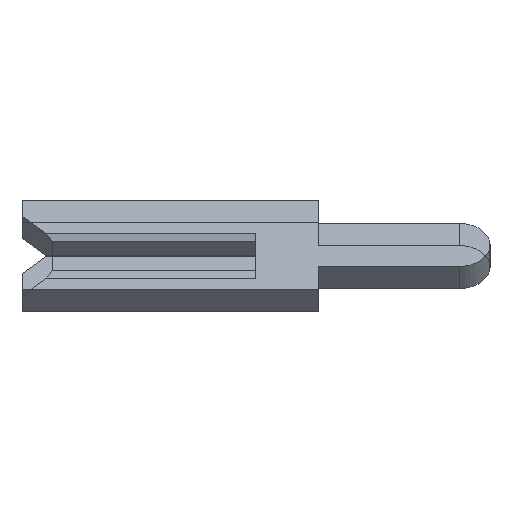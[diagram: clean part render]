
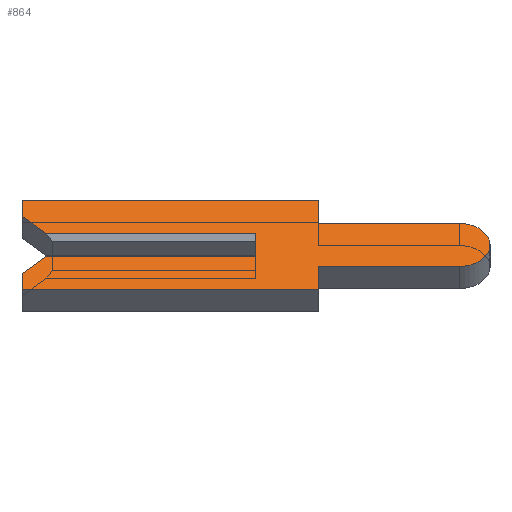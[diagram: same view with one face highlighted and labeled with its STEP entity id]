
A CAD part, left-side view. The second image highlights one B-rep face of the part: STEP entity #864.
In plain terms, the highlighted face is planar.
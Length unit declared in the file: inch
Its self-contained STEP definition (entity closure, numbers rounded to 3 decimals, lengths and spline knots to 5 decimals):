
#9 = CARTESIAN_POINT ( 'NONE',  ( -0.01, -0.1305, 0. ) ) ;
#24 = DIRECTION ( 'NONE',  ( 0., 0., -1. ) ) ;
#28 = VERTEX_POINT ( 'NONE', #462 ) ;
#91 = EDGE_CURVE ( 'NONE', #2926, #1471, #1673, .T. ) ;
#92 = CARTESIAN_POINT ( 'NONE',  ( -0.01, -0.04, 0.0195 ) ) ;
#119 = VECTOR ( 'NONE', #1464, 39.37008 ) ;
#138 = VECTOR ( 'NONE', #2182, 39.37008 ) ;
#164 = EDGE_CURVE ( 'NONE', #231, #1471, #1262, .T. ) ;
#183 = CARTESIAN_POINT ( 'NONE',  ( -0.01, 0.1305, -0.0065 ) ) ;
#231 = VERTEX_POINT ( 'NONE', #2669 ) ;
#281 = VERTEX_POINT ( 'NONE', #2938 ) ;
#291 = FACE_OUTER_BOUND ( 'NONE', #2627, .T. ) ;
#386 = ORIENTED_EDGE ( 'NONE', *, *, #2870, .F. ) ;
#456 = CARTESIAN_POINT ( 'NONE',  ( -0.01, 0.15, -0.026 ) ) ;
#462 = CARTESIAN_POINT ( 'NONE',  ( -0.01, -0.04, -0.0195 ) ) ;
#463 = EDGE_CURVE ( 'NONE', #2926, #2965, #843, .T. ) ;
#465 = VECTOR ( 'NONE', #735, 39.37008 ) ;
#523 = CARTESIAN_POINT ( 'NONE',  ( -0.01, 0., 0.0065 ) ) ;
#561 = DIRECTION ( 'NONE',  ( 1., 0., 0. ) ) ;
#573 = CARTESIAN_POINT ( 'NONE',  ( -0.01, -0.04, -0.04 ) ) ;
#591 = VECTOR ( 'NONE', #1389, 39.37008 ) ;
#613 = ORIENTED_EDGE ( 'NONE', *, *, #886, .F. ) ;
#616 = AXIS2_PLACEMENT_3D ( 'NONE', #9, #561, #24 ) ;
#646 = DIRECTION ( 'NONE',  ( 0., 0., -1. ) ) ;
#657 = CARTESIAN_POINT ( 'NONE',  ( -0.01, -0.1305, 0. ) ) ;
#684 = VERTEX_POINT ( 'NONE', #2724 ) ;
#710 = EDGE_CURVE ( 'NONE', #684, #231, #763, .T. ) ;
#728 = DIRECTION ( 'NONE',  ( 0., 0., 1. ) ) ;
#735 = DIRECTION ( 'NONE',  ( 0., -0.707, 0.707 ) ) ;
#763 = LINE ( 'NONE', #1929, #591 ) ;
#774 = ORIENTED_EDGE ( 'NONE', *, *, #2505, .F. ) ;
#800 = EDGE_CURVE ( 'NONE', #2965, #935, #2738, .T. ) ;
#820 = ORIENTED_EDGE ( 'NONE', *, *, #91, .T. ) ;
#829 = DIRECTION ( 'NONE',  ( 0., -1., 0. ) ) ;
#843 = LINE ( 'NONE', #2047, #138 ) ;
#864 = ADVANCED_FACE ( 'NONE', ( #291 ), #1636, .F. ) ;
#869 = VECTOR ( 'NONE', #1067, 39.37008 ) ;
#886 = EDGE_CURVE ( 'NONE', #1972, #3171, #2114, .T. ) ;
#935 = VERTEX_POINT ( 'NONE', #3116 ) ;
#1065 = VERTEX_POINT ( 'NONE', #3326 ) ;
#1067 = DIRECTION ( 'NONE',  ( 0., -1., 0. ) ) ;
#1164 = DIRECTION ( 'NONE',  ( 0., -1., 0. ) ) ;
#1177 = LINE ( 'NONE', #183, #465 ) ;
#1187 = EDGE_CURVE ( 'NONE', #28, #1530, #1839, .T. ) ;
#1262 = LINE ( 'NONE', #523, #1321 ) ;
#1277 = ORIENTED_EDGE ( 'NONE', *, *, #2949, .F. ) ;
#1303 = ORIENTED_EDGE ( 'NONE', *, *, #164, .F. ) ;
#1321 = VECTOR ( 'NONE', #1600, 39.37008 ) ;
#1327 = CARTESIAN_POINT ( 'NONE',  ( -0.01, 0.15, 0.01 ) ) ;
#1375 = CARTESIAN_POINT ( 'NONE',  ( -0.01, 0.15, 0.026 ) ) ;
#1389 = DIRECTION ( 'NONE',  ( 0., -1., 0. ) ) ;
#1464 = DIRECTION ( 'NONE',  ( 0., 1., 0. ) ) ;
#1471 = VERTEX_POINT ( 'NONE', #2883 ) ;
#1485 = ORIENTED_EDGE ( 'NONE', *, *, #1187, .F. ) ;
#1530 = VERTEX_POINT ( 'NONE', #2732 ) ;
#1557 = LINE ( 'NONE', #2789, #119 ) ;
#1561 = ORIENTED_EDGE ( 'NONE', *, *, #800, .F. ) ;
#1564 = CARTESIAN_POINT ( 'NONE',  ( -0.01, -0.1305, -0.0195 ) ) ;
#1573 = VECTOR ( 'NONE', #3124, 39.37008 ) ;
#1582 = LINE ( 'NONE', #456, #3179 ) ;
#1589 = VERTEX_POINT ( 'NONE', #1564 ) ;
#1600 = DIRECTION ( 'NONE',  ( 0., 0., 1. ) ) ;
#1636 = PLANE ( 'NONE',  #616 ) ;
#1673 = LINE ( 'NONE', #1327, #869 ) ;
#1768 = LINE ( 'NONE', #3133, #3098 ) ;
#1804 = EDGE_CURVE ( 'NONE', #281, #684, #1177, .T. ) ;
#1831 = ORIENTED_EDGE ( 'NONE', *, *, #2131, .F. ) ;
#1839 = LINE ( 'NONE', #573, #1573 ) ;
#1842 = VERTEX_POINT ( 'NONE', #2617 ) ;
#1852 = LINE ( 'NONE', #3298, #3362 ) ;
#1881 = CIRCLE ( 'NONE', #2850, 0.0195 ) ;
#1889 = EDGE_CURVE ( 'NONE', #3171, #1589, #1881, .T. ) ;
#1908 = CARTESIAN_POINT ( 'NONE',  ( -0.01, -0.04, 0.0195 ) ) ;
#1929 = CARTESIAN_POINT ( 'NONE',  ( -0.01, -0.1305, -0.01 ) ) ;
#1972 = VERTEX_POINT ( 'NONE', #92 ) ;
#2011 = CARTESIAN_POINT ( 'NONE',  ( -0.01, -0.1305, 0.0195 ) ) ;
#2047 = CARTESIAN_POINT ( 'NONE',  ( -0.01, 0.1305, 0.0065 ) ) ;
#2048 = ORIENTED_EDGE ( 'NONE', *, *, #463, .F. ) ;
#2094 = ORIENTED_EDGE ( 'NONE', *, *, #1889, .F. ) ;
#2114 = LINE ( 'NONE', #1908, #2187 ) ;
#2131 = EDGE_CURVE ( 'NONE', #1530, #1065, #1557, .T. ) ;
#2182 = DIRECTION ( 'NONE',  ( 0., 0.707, 0.707 ) ) ;
#2187 = VECTOR ( 'NONE', #829, 39.37008 ) ;
#2246 = DIRECTION ( 'NONE',  ( 1., 0., 0. ) ) ;
#2254 = CARTESIAN_POINT ( 'NONE',  ( -0.01, -0.04, 0.04 ) ) ;
#2259 = DIRECTION ( 'NONE',  ( 0., 0., -1. ) ) ;
#2440 = DIRECTION ( 'NONE',  ( 0., 0., 1. ) ) ;
#2442 = ORIENTED_EDGE ( 'NONE', *, *, #710, .F. ) ;
#2458 = LINE ( 'NONE', #2254, #3257 ) ;
#2505 = EDGE_CURVE ( 'NONE', #935, #1842, #1852, .T. ) ;
#2617 = CARTESIAN_POINT ( 'NONE',  ( -0.01, -0.04, 0.04 ) ) ;
#2627 = EDGE_LOOP ( 'NONE', ( #820, #1303, #2442, #3343, #1277, #1831, #1485, #3007, #2094, #613, #386, #774, #1561, #2048 ) ) ;
#2669 = CARTESIAN_POINT ( 'NONE',  ( -0.01, 0., -0.01 ) ) ;
#2724 = CARTESIAN_POINT ( 'NONE',  ( -0.01, 0.134, -0.01 ) ) ;
#2732 = CARTESIAN_POINT ( 'NONE',  ( -0.01, -0.04, -0.04 ) ) ;
#2738 = LINE ( 'NONE', #1375, #3232 ) ;
#2789 = CARTESIAN_POINT ( 'NONE',  ( -0.01, 0.15, -0.04 ) ) ;
#2791 = CARTESIAN_POINT ( 'NONE',  ( -0.01, 0.15, 0.026 ) ) ;
#2850 = AXIS2_PLACEMENT_3D ( 'NONE', #657, #2246, #2259 ) ;
#2870 = EDGE_CURVE ( 'NONE', #1842, #1972, #2458, .T. ) ;
#2873 = DIRECTION ( 'NONE',  ( 0., 1., 0. ) ) ;
#2883 = CARTESIAN_POINT ( 'NONE',  ( -0.01, 0., 0.01 ) ) ;
#2926 = VERTEX_POINT ( 'NONE', #3067 ) ;
#2938 = CARTESIAN_POINT ( 'NONE',  ( -0.01, 0.15, -0.026 ) ) ;
#2949 = EDGE_CURVE ( 'NONE', #1065, #281, #1582, .T. ) ;
#2965 = VERTEX_POINT ( 'NONE', #2791 ) ;
#3007 = ORIENTED_EDGE ( 'NONE', *, *, #3031, .F. ) ;
#3031 = EDGE_CURVE ( 'NONE', #1589, #28, #1768, .T. ) ;
#3067 = CARTESIAN_POINT ( 'NONE',  ( -0.01, 0.134, 0.01 ) ) ;
#3098 = VECTOR ( 'NONE', #2873, 39.37008 ) ;
#3116 = CARTESIAN_POINT ( 'NONE',  ( -0.01, 0.15, 0.04 ) ) ;
#3124 = DIRECTION ( 'NONE',  ( 0., 0., -1. ) ) ;
#3133 = CARTESIAN_POINT ( 'NONE',  ( -0.01, -0.04, -0.0195 ) ) ;
#3171 = VERTEX_POINT ( 'NONE', #2011 ) ;
#3179 = VECTOR ( 'NONE', #728, 39.37008 ) ;
#3232 = VECTOR ( 'NONE', #2440, 39.37008 ) ;
#3257 = VECTOR ( 'NONE', #646, 39.37008 ) ;
#3298 = CARTESIAN_POINT ( 'NONE',  ( -0.01, 0.15, 0.04 ) ) ;
#3326 = CARTESIAN_POINT ( 'NONE',  ( -0.01, 0.15, -0.04 ) ) ;
#3343 = ORIENTED_EDGE ( 'NONE', *, *, #1804, .F. ) ;
#3362 = VECTOR ( 'NONE', #1164, 39.37008 ) ;
